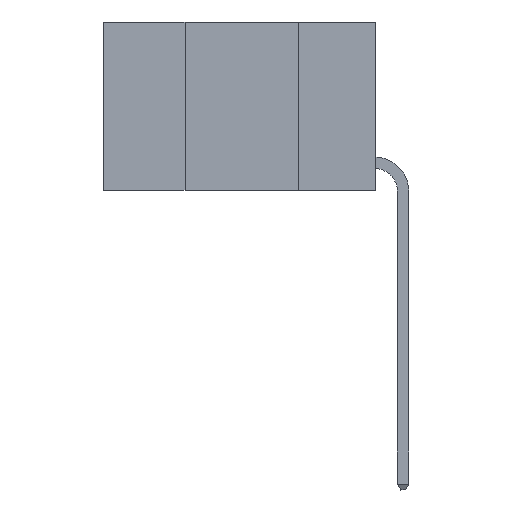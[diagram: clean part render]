
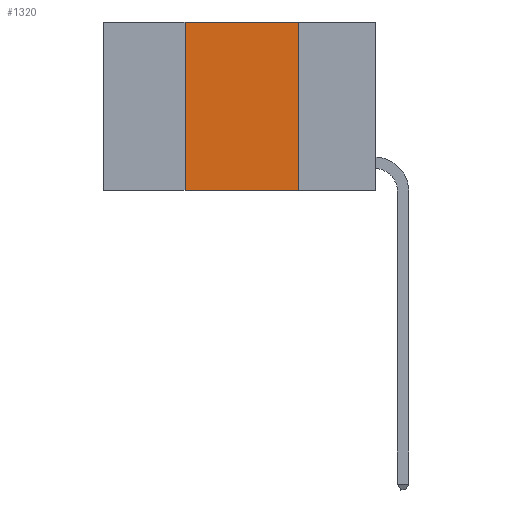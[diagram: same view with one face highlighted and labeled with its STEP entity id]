
A CAD part, left-side view. The second image highlights one B-rep face of the part: STEP entity #1320.
In plain terms, the highlighted planar face has unit normal (-1, 0, 0).
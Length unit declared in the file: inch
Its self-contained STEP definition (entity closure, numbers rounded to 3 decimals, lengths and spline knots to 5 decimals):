
#78 = VERTEX_POINT ( 'NONE', #1648 ) ;
#108 = VECTOR ( 'NONE', #6492, 39.37008 ) ;
#356 = ORIENTED_EDGE ( 'NONE', *, *, #9628, .F. ) ;
#1166 = VECTOR ( 'NONE', #10452, 39.37008 ) ;
#1264 = ORIENTED_EDGE ( 'NONE', *, *, #6349, .T. ) ;
#1320 = ADVANCED_FACE ( 'NONE', ( #2467 ), #1653, .F. ) ;
#1389 = CARTESIAN_POINT ( 'NONE',  ( 0., 0.6, 0. ) ) ;
#1648 = CARTESIAN_POINT ( 'NONE',  ( 0., 0.42, 0. ) ) ;
#1653 = PLANE ( 'NONE',  #2610 ) ;
#1960 = ORIENTED_EDGE ( 'NONE', *, *, #6631, .F. ) ;
#2003 = LINE ( 'NONE', #8669, #5761 ) ;
#2467 = FACE_OUTER_BOUND ( 'NONE', #7280, .T. ) ;
#2610 = AXIS2_PLACEMENT_3D ( 'NONE', #4978, #4174, #7490 ) ;
#3609 = VERTEX_POINT ( 'NONE', #10086 ) ;
#3940 = EDGE_CURVE ( 'NONE', #3609, #10463, #9826, .T. ) ;
#4174 = DIRECTION ( 'NONE',  ( 1., 0., 0. ) ) ;
#4459 = DIRECTION ( 'NONE',  ( 0., 0., 1. ) ) ;
#4712 = LINE ( 'NONE', #1389, #108 ) ;
#4978 = CARTESIAN_POINT ( 'NONE',  ( 0., 0.6, 0. ) ) ;
#5761 = VECTOR ( 'NONE', #6186, 39.37008 ) ;
#6186 = DIRECTION ( 'NONE',  ( 0., -1., 0. ) ) ;
#6227 = CARTESIAN_POINT ( 'NONE',  ( 0., 0.42, 0. ) ) ;
#6349 = EDGE_CURVE ( 'NONE', #8041, #10463, #2003, .T. ) ;
#6492 = DIRECTION ( 'NONE',  ( 0., -1., 0. ) ) ;
#6631 = EDGE_CURVE ( 'NONE', #8041, #78, #9459, .T. ) ;
#7280 = EDGE_LOOP ( 'NONE', ( #8417, #356, #1960, #1264 ) ) ;
#7490 = DIRECTION ( 'NONE',  ( 0., 0., -1. ) ) ;
#8041 = VERTEX_POINT ( 'NONE', #10158 ) ;
#8417 = ORIENTED_EDGE ( 'NONE', *, *, #3940, .F. ) ;
#8669 = CARTESIAN_POINT ( 'NONE',  ( 0., 0.6, -0.37 ) ) ;
#8755 = VECTOR ( 'NONE', #4459, 39.37008 ) ;
#9459 = LINE ( 'NONE', #6227, #8755 ) ;
#9628 = EDGE_CURVE ( 'NONE', #78, #3609, #4712, .T. ) ;
#9826 = LINE ( 'NONE', #10602, #1166 ) ;
#9915 = CARTESIAN_POINT ( 'NONE',  ( 0., 0.17, -0.37 ) ) ;
#10086 = CARTESIAN_POINT ( 'NONE',  ( 0., 0.17, 0. ) ) ;
#10158 = CARTESIAN_POINT ( 'NONE',  ( 0., 0.42, -0.37 ) ) ;
#10452 = DIRECTION ( 'NONE',  ( 0., 0., -1. ) ) ;
#10463 = VERTEX_POINT ( 'NONE', #9915 ) ;
#10602 = CARTESIAN_POINT ( 'NONE',  ( 0., 0.17, 0. ) ) ;
